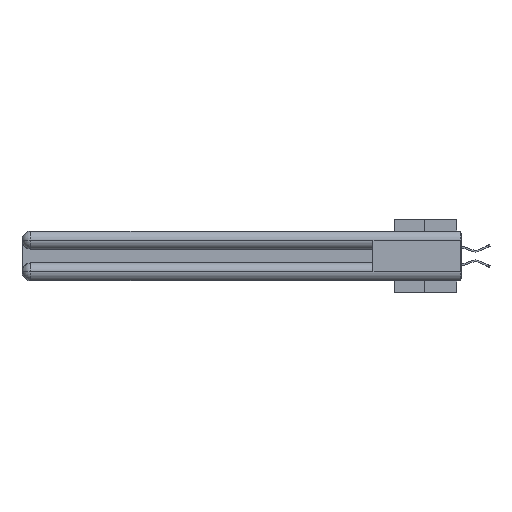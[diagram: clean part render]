
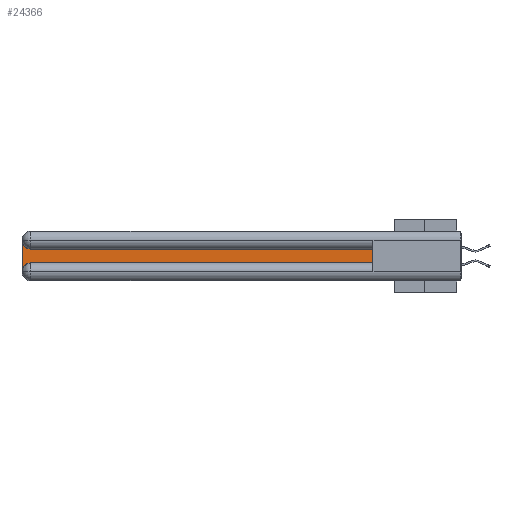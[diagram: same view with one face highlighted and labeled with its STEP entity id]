
A CAD part, left-side view. The second image highlights one B-rep face of the part: STEP entity #24366.
In plain terms, the highlighted planar face has unit normal (-1, 0, 0).
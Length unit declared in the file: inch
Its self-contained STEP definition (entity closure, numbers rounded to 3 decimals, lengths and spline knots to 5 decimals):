
#302 = ORIENTED_EDGE ( 'NONE', *, *, #9977, .T. ) ;
#943 = AXIS2_PLACEMENT_3D ( 'NONE', #35676, #21496, #35828 ) ;
#1426 = EDGE_CURVE ( 'NONE', #11043, #21859, #2749, .T. ) ;
#1702 = ORIENTED_EDGE ( 'NONE', *, *, #23157, .T. ) ;
#2749 = LINE ( 'NONE', #6782, #25097 ) ;
#6782 = CARTESIAN_POINT ( 'NONE',  ( 0.075, 0.6, -0.2175 ) ) ;
#7872 = EDGE_LOOP ( 'NONE', ( #29676, #26527, #1702, #38145, #13593, #302 ) ) ;
#9379 = CARTESIAN_POINT ( 'NONE',  ( 0.075, 3., -0.0625 ) ) ;
#9450 = VERTEX_POINT ( 'NONE', #9379 ) ;
#9977 = EDGE_CURVE ( 'NONE', #21859, #41448, #22275, .T. ) ;
#11043 = VERTEX_POINT ( 'NONE', #30457 ) ;
#12928 = EDGE_CURVE ( 'NONE', #41448, #46828, #43164, .T. ) ;
#13081 = DIRECTION ( 'NONE',  ( 1., 0., 0. ) ) ;
#13593 = ORIENTED_EDGE ( 'NONE', *, *, #1426, .T. ) ;
#15070 = LINE ( 'NONE', #45473, #16827 ) ;
#16827 = VECTOR ( 'NONE', #28240, 39.37008 ) ;
#17326 = DIRECTION ( 'NONE',  ( 0., 1., 0. ) ) ;
#17352 = PLANE ( 'NONE',  #943 ) ;
#20152 = FACE_OUTER_BOUND ( 'NONE', #7872, .T. ) ;
#20735 = CARTESIAN_POINT ( 'NONE',  ( 0.075, 0.6, -0.2175 ) ) ;
#21496 = DIRECTION ( 'NONE',  ( 1., 0., 0. ) ) ;
#21859 = VERTEX_POINT ( 'NONE', #40926 ) ;
#22028 = CARTESIAN_POINT ( 'NONE',  ( 0.075, 3., -0.2775 ) ) ;
#22275 = LINE ( 'NONE', #20735, #45153 ) ;
#23157 = EDGE_CURVE ( 'NONE', #9450, #41036, #15070, .T. ) ;
#23260 = CARTESIAN_POINT ( 'NONE',  ( 0.075, 2.94, -0.2775 ) ) ;
#24000 = CIRCLE ( 'NONE', #40793, 0.06 ) ;
#24366 = ADVANCED_FACE ( 'NONE', ( #20152 ), #17352, .F. ) ;
#25097 = VECTOR ( 'NONE', #32506, 39.37008 ) ;
#25666 = EDGE_CURVE ( 'NONE', #46828, #9450, #24000, .T. ) ;
#26358 = EDGE_CURVE ( 'NONE', #41036, #11043, #39320, .T. ) ;
#26527 = ORIENTED_EDGE ( 'NONE', *, *, #25666, .T. ) ;
#26979 = CARTESIAN_POINT ( 'NONE',  ( 0.075, 0.6, -0.1225 ) ) ;
#28240 = DIRECTION ( 'NONE',  ( 0., 0., -1. ) ) ;
#29676 = ORIENTED_EDGE ( 'NONE', *, *, #12928, .T. ) ;
#30457 = CARTESIAN_POINT ( 'NONE',  ( 0.075, 2.94, -0.2175 ) ) ;
#30905 = DIRECTION ( 'NONE',  ( 0., 0., -1. ) ) ;
#32506 = DIRECTION ( 'NONE',  ( 0., -1., 0. ) ) ;
#33426 = VECTOR ( 'NONE', #17326, 39.37008 ) ;
#33611 = CARTESIAN_POINT ( 'NONE',  ( 0.075, 0.6, -0.1225 ) ) ;
#35076 = DIRECTION ( 'NONE',  ( 0., 0., 1. ) ) ;
#35676 = CARTESIAN_POINT ( 'NONE',  ( 0.075, 3., -0.1225 ) ) ;
#35828 = DIRECTION ( 'NONE',  ( 0., 0., -1. ) ) ;
#38145 = ORIENTED_EDGE ( 'NONE', *, *, #26358, .T. ) ;
#39320 = CIRCLE ( 'NONE', #43836, 0.06 ) ;
#40793 = AXIS2_PLACEMENT_3D ( 'NONE', #42034, #13081, #45663 ) ;
#40926 = CARTESIAN_POINT ( 'NONE',  ( 0.075, 0.6, -0.2175 ) ) ;
#41036 = VERTEX_POINT ( 'NONE', #22028 ) ;
#41339 = DIRECTION ( 'NONE',  ( 1., 0., 0. ) ) ;
#41448 = VERTEX_POINT ( 'NONE', #33611 ) ;
#42034 = CARTESIAN_POINT ( 'NONE',  ( 0.075, 2.94, -0.0625 ) ) ;
#43070 = CARTESIAN_POINT ( 'NONE',  ( 0.075, 2.94, -0.1225 ) ) ;
#43164 = LINE ( 'NONE', #26979, #33426 ) ;
#43836 = AXIS2_PLACEMENT_3D ( 'NONE', #23260, #41339, #30905 ) ;
#45153 = VECTOR ( 'NONE', #35076, 39.37008 ) ;
#45473 = CARTESIAN_POINT ( 'NONE',  ( 0.075, 3., -0.2175 ) ) ;
#45663 = DIRECTION ( 'NONE',  ( 0., 0., -1. ) ) ;
#46828 = VERTEX_POINT ( 'NONE', #43070 ) ;
